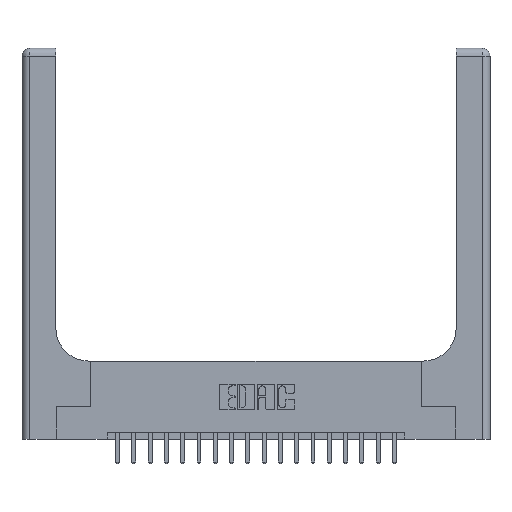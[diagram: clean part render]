
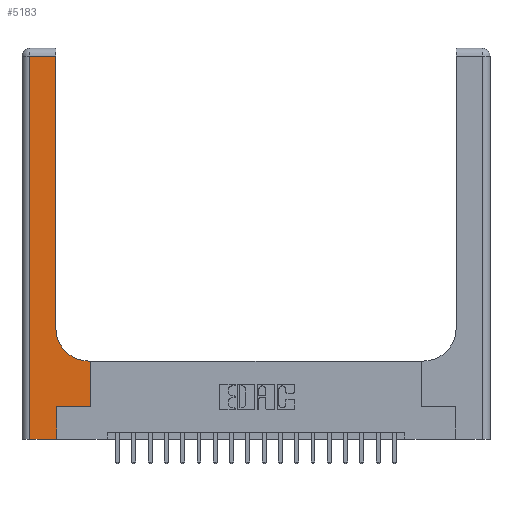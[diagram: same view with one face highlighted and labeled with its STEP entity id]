
A CAD part, top view. The second image highlights one B-rep face of the part: STEP entity #5183.
In plain terms, the highlighted planar face has unit normal (0, 0, 1).
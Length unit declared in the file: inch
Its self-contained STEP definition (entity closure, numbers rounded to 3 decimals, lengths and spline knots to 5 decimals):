
#37 = CIRCLE ( 'NONE', #12562, 0.25 ) ;
#104 = CARTESIAN_POINT ( 'NONE',  ( 0.265, 0.25, 0.37 ) ) ;
#366 = EDGE_CURVE ( 'NONE', #20163, #1574, #11418, .T. ) ;
#464 = CARTESIAN_POINT ( 'NONE',  ( 0.26, 0.6, 0.37 ) ) ;
#876 = EDGE_CURVE ( 'NONE', #1574, #17392, #4786, .T. ) ;
#882 = VERTEX_POINT ( 'NONE', #16157 ) ;
#1056 = CARTESIAN_POINT ( 'NONE',  ( 0., 3., 0.37 ) ) ;
#1140 = ORIENTED_EDGE ( 'NONE', *, *, #5870, .T. ) ;
#1187 = CARTESIAN_POINT ( 'NONE',  ( 0.265, 0., 0.37 ) ) ;
#1221 = DIRECTION ( 'NONE',  ( 0., 0., -1. ) ) ;
#1323 = VECTOR ( 'NONE', #8397, 39.37008 ) ;
#1530 = VECTOR ( 'NONE', #7789, 39.37008 ) ;
#1574 = VERTEX_POINT ( 'NONE', #7285 ) ;
#2060 = CARTESIAN_POINT ( 'NONE',  ( 0., 2.94, 0.37 ) ) ;
#3141 = EDGE_CURVE ( 'NONE', #12409, #20163, #37, .T. ) ;
#3743 = LINE ( 'NONE', #3995, #1530 ) ;
#3953 = CARTESIAN_POINT ( 'NONE',  ( 0.51, 0.6, 0.37 ) ) ;
#3979 = DIRECTION ( 'NONE',  ( 1., 0., 0. ) ) ;
#3995 = CARTESIAN_POINT ( 'NONE',  ( 0., 0., 0.37 ) ) ;
#4064 = VECTOR ( 'NONE', #20198, 39.37008 ) ;
#4553 = DIRECTION ( 'NONE',  ( 0., 1., 0. ) ) ;
#4576 = LINE ( 'NONE', #1187, #12156 ) ;
#4786 = LINE ( 'NONE', #2060, #1323 ) ;
#4910 = ORIENTED_EDGE ( 'NONE', *, *, #3141, .T. ) ;
#5068 = VERTEX_POINT ( 'NONE', #15733 ) ;
#5183 = ADVANCED_FACE ( 'NONE', ( #6266 ), #17969, .F. ) ;
#5220 = VECTOR ( 'NONE', #4553, 39.37008 ) ;
#5244 = DIRECTION ( 'NONE',  ( -1., 0., 0. ) ) ;
#5870 = EDGE_CURVE ( 'NONE', #17678, #20160, #12836, .T. ) ;
#6266 = FACE_OUTER_BOUND ( 'NONE', #11916, .T. ) ;
#6514 = EDGE_CURVE ( 'NONE', #882, #5068, #3743, .T. ) ;
#6959 = ORIENTED_EDGE ( 'NONE', *, *, #876, .T. ) ;
#7001 = ORIENTED_EDGE ( 'NONE', *, *, #366, .T. ) ;
#7285 = CARTESIAN_POINT ( 'NONE',  ( 0.26, 2.94, 0.37 ) ) ;
#7481 = CARTESIAN_POINT ( 'NONE',  ( 0.26, 3., 0.37 ) ) ;
#7628 = CARTESIAN_POINT ( 'NONE',  ( 0.528, 0.25, 0.37 ) ) ;
#7654 = DIRECTION ( 'NONE',  ( 0., 1., 0. ) ) ;
#7656 = EDGE_CURVE ( 'NONE', #20160, #19627, #15476, .T. ) ;
#7789 = DIRECTION ( 'NONE',  ( 1., 0., 0. ) ) ;
#8279 = CARTESIAN_POINT ( 'NONE',  ( 0.528, 0.6, 0.37 ) ) ;
#8397 = DIRECTION ( 'NONE',  ( -1., 0., 0. ) ) ;
#8714 = LINE ( 'NONE', #464, #13827 ) ;
#8774 = ORIENTED_EDGE ( 'NONE', *, *, #17051, .T. ) ;
#8951 = DIRECTION ( 'NONE',  ( 1., 0., 0. ) ) ;
#9364 = CARTESIAN_POINT ( 'NONE',  ( 0.26, 0.85, 0.37 ) ) ;
#10635 = ORIENTED_EDGE ( 'NONE', *, *, #19453, .T. ) ;
#11318 = ORIENTED_EDGE ( 'NONE', *, *, #7656, .T. ) ;
#11418 = LINE ( 'NONE', #7481, #4064 ) ;
#11916 = EDGE_LOOP ( 'NONE', ( #7001, #6959, #16740, #17326, #10635, #1140, #11318, #8774, #4910 ) ) ;
#12130 = CARTESIAN_POINT ( 'NONE',  ( 0.06, 2.94, 0.37 ) ) ;
#12156 = VECTOR ( 'NONE', #7654, 39.37008 ) ;
#12409 = VERTEX_POINT ( 'NONE', #3953 ) ;
#12562 = AXIS2_PLACEMENT_3D ( 'NONE', #18419, #1221, #8951 ) ;
#12712 = AXIS2_PLACEMENT_3D ( 'NONE', #1056, #13714, #18305 ) ;
#12836 = LINE ( 'NONE', #13342, #15515 ) ;
#12998 = VECTOR ( 'NONE', #14963, 39.37008 ) ;
#13342 = CARTESIAN_POINT ( 'NONE',  ( 0.265, 0.25, 0.37 ) ) ;
#13714 = DIRECTION ( 'NONE',  ( 0., 0., -1. ) ) ;
#13722 = EDGE_CURVE ( 'NONE', #17392, #882, #19119, .T. ) ;
#13827 = VECTOR ( 'NONE', #5244, 39.37008 ) ;
#14963 = DIRECTION ( 'NONE',  ( 0., -1., 0. ) ) ;
#15476 = LINE ( 'NONE', #7628, #5220 ) ;
#15480 = CARTESIAN_POINT ( 'NONE',  ( 0.528, 0.25, 0.37 ) ) ;
#15515 = VECTOR ( 'NONE', #3979, 39.37008 ) ;
#15733 = CARTESIAN_POINT ( 'NONE',  ( 0.265, 0., 0.37 ) ) ;
#16157 = CARTESIAN_POINT ( 'NONE',  ( 0.06, 0., 0.37 ) ) ;
#16740 = ORIENTED_EDGE ( 'NONE', *, *, #13722, .T. ) ;
#17051 = EDGE_CURVE ( 'NONE', #19627, #12409, #8714, .T. ) ;
#17326 = ORIENTED_EDGE ( 'NONE', *, *, #6514, .T. ) ;
#17392 = VERTEX_POINT ( 'NONE', #12130 ) ;
#17678 = VERTEX_POINT ( 'NONE', #104 ) ;
#17969 = PLANE ( 'NONE',  #12712 ) ;
#18305 = DIRECTION ( 'NONE',  ( -1., 0., 0. ) ) ;
#18419 = CARTESIAN_POINT ( 'NONE',  ( 0.51, 0.85, 0.37 ) ) ;
#19119 = LINE ( 'NONE', #19846, #12998 ) ;
#19453 = EDGE_CURVE ( 'NONE', #5068, #17678, #4576, .T. ) ;
#19627 = VERTEX_POINT ( 'NONE', #8279 ) ;
#19846 = CARTESIAN_POINT ( 'NONE',  ( 0.06, 3., 0.37 ) ) ;
#20160 = VERTEX_POINT ( 'NONE', #15480 ) ;
#20163 = VERTEX_POINT ( 'NONE', #9364 ) ;
#20198 = DIRECTION ( 'NONE',  ( 0., 1., 0. ) ) ;
